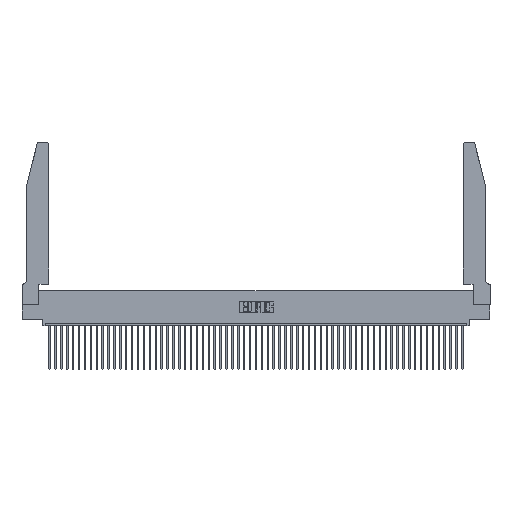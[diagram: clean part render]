
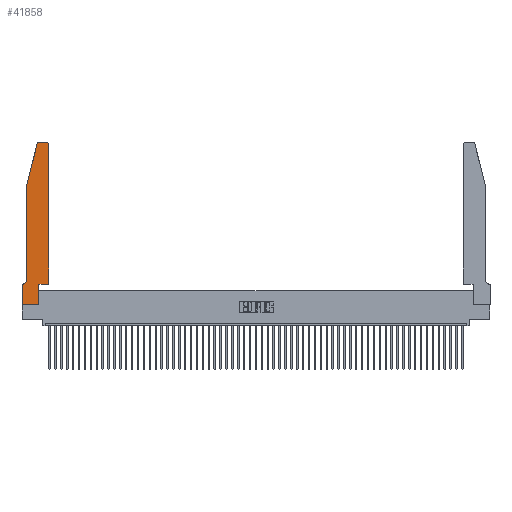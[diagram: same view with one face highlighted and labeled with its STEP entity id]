
A CAD part, top view. The second image highlights one B-rep face of the part: STEP entity #41858.
In plain terms, the highlighted planar face has unit normal (0, 0, 1).
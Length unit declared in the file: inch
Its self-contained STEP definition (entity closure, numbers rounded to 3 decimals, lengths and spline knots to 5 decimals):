
#1388 = CARTESIAN_POINT ( 'NONE',  ( 0.4505, 0.35, 0.37 ) ) ;
#1948 = DIRECTION ( 'NONE',  ( 0., 0., 1. ) ) ;
#2347 = CARTESIAN_POINT ( 'NONE',  ( 0., 0.35, 0.37 ) ) ;
#2770 = DIRECTION ( 'NONE',  ( 0., -1., 0. ) ) ;
#3745 = EDGE_CURVE ( 'NONE', #12074, #40353, #35902, .T. ) ;
#3822 = EDGE_LOOP ( 'NONE', ( #51862, #30141, #5879, #22489, #43303, #23899, #53336, #4882, #50175, #13437, #8664, #28840 ) ) ;
#4216 = DIRECTION ( 'NONE',  ( -0.239, -0.971, 0. ) ) ;
#4882 = ORIENTED_EDGE ( 'NONE', *, *, #9215, .T. ) ;
#5189 = LINE ( 'NONE', #21240, #26146 ) ;
#5588 = DIRECTION ( 'NONE',  ( -1., 0., 0. ) ) ;
#5879 = ORIENTED_EDGE ( 'NONE', *, *, #35239, .T. ) ;
#6450 = DIRECTION ( 'NONE',  ( -1., 0., 0. ) ) ;
#7061 = CARTESIAN_POINT ( 'NONE',  ( 0., 0., 0.37 ) ) ;
#8207 = LINE ( 'NONE', #7061, #25242 ) ;
#8257 = CIRCLE ( 'NONE', #15924, 0.07 ) ;
#8345 = CARTESIAN_POINT ( 'NONE',  ( 0.2605, 2.75, 0.37 ) ) ;
#8349 = CARTESIAN_POINT ( 'NONE',  ( 0.0755, 2., 0.37 ) ) ;
#8664 = ORIENTED_EDGE ( 'NONE', *, *, #11363, .T. ) ;
#9215 = EDGE_CURVE ( 'NONE', #18021, #46392, #42642, .T. ) ;
#9632 = DIRECTION ( 'NONE',  ( -1., 0., 0. ) ) ;
#10883 = VECTOR ( 'NONE', #48942, 39.37008 ) ;
#11363 = EDGE_CURVE ( 'NONE', #18905, #37915, #25783, .T. ) ;
#11902 = FACE_OUTER_BOUND ( 'NONE', #3822, .T. ) ;
#12074 = VERTEX_POINT ( 'NONE', #8349 ) ;
#13437 = ORIENTED_EDGE ( 'NONE', *, *, #32538, .T. ) ;
#13630 = CARTESIAN_POINT ( 'NONE',  ( 0.0055, 0.35, 0.37 ) ) ;
#13858 = DIRECTION ( 'NONE',  ( 0., 0., -1. ) ) ;
#15619 = AXIS2_PLACEMENT_3D ( 'NONE', #2347, #1948, #40471 ) ;
#15924 = AXIS2_PLACEMENT_3D ( 'NONE', #34773, #13858, #9632 ) ;
#18021 = VERTEX_POINT ( 'NONE', #51473 ) ;
#18905 = VERTEX_POINT ( 'NONE', #1388 ) ;
#19006 = CARTESIAN_POINT ( 'NONE',  ( 0.284, 2.75, 0.37 ) ) ;
#19090 = CARTESIAN_POINT ( 'NONE',  ( 0.0755, 0.35, 0.37 ) ) ;
#19500 = VERTEX_POINT ( 'NONE', #28431 ) ;
#20031 = EDGE_CURVE ( 'NONE', #39617, #21007, #28667, .T. ) ;
#20418 = DIRECTION ( 'NONE',  ( 1., 0., 0. ) ) ;
#20900 = VECTOR ( 'NONE', #33370, 39.37008 ) ;
#21007 = VERTEX_POINT ( 'NONE', #31247 ) ;
#21132 = CIRCLE ( 'NONE', #23765, 0.03 ) ;
#21152 = VERTEX_POINT ( 'NONE', #13630 ) ;
#21240 = CARTESIAN_POINT ( 'NONE',  ( 0.0755, 2., 0.37 ) ) ;
#21683 = EDGE_CURVE ( 'NONE', #19500, #18021, #8207, .T. ) ;
#22460 = CARTESIAN_POINT ( 'NONE',  ( 0.2865, 0.35, 0.37 ) ) ;
#22489 = ORIENTED_EDGE ( 'NONE', *, *, #3745, .T. ) ;
#22784 = LINE ( 'NONE', #22460, #52374 ) ;
#23283 = DIRECTION ( 'NONE',  ( 0., 1., 0. ) ) ;
#23765 = AXIS2_PLACEMENT_3D ( 'NONE', #37857, #33274, #20418 ) ;
#23769 = CARTESIAN_POINT ( 'NONE',  ( 0.2865, 0.35, 0.37 ) ) ;
#23899 = ORIENTED_EDGE ( 'NONE', *, *, #48974, .T. ) ;
#25242 = VECTOR ( 'NONE', #2770, 39.37008 ) ;
#25735 = LINE ( 'NONE', #8345, #48185 ) ;
#25783 = LINE ( 'NONE', #36173, #34985 ) ;
#26146 = VECTOR ( 'NONE', #4216, 39.37008 ) ;
#26509 = VECTOR ( 'NONE', #6450, 39.37008 ) ;
#26691 = CARTESIAN_POINT ( 'NONE',  ( 0.4205, 2.75, 0.37 ) ) ;
#28431 = CARTESIAN_POINT ( 'NONE',  ( 0., 0.35, 0.37 ) ) ;
#28667 = CIRCLE ( 'NONE', #48745, 0.03 ) ;
#28755 = VERTEX_POINT ( 'NONE', #26691 ) ;
#28840 = ORIENTED_EDGE ( 'NONE', *, *, #46699, .T. ) ;
#29139 = EDGE_CURVE ( 'NONE', #40353, #21152, #8257, .T. ) ;
#29727 = EDGE_CURVE ( 'NONE', #28755, #39617, #25735, .T. ) ;
#30047 = DIRECTION ( 'NONE',  ( 1., 0., 0. ) ) ;
#30141 = ORIENTED_EDGE ( 'NONE', *, *, #20031, .T. ) ;
#30896 = CARTESIAN_POINT ( 'NONE',  ( 0.284, 2.72, 0.37 ) ) ;
#31247 = CARTESIAN_POINT ( 'NONE',  ( 0.25487, 2.72718, 0.37 ) ) ;
#31370 = LINE ( 'NONE', #38742, #42628 ) ;
#32538 = EDGE_CURVE ( 'NONE', #52554, #18905, #31370, .T. ) ;
#32606 = CARTESIAN_POINT ( 'NONE',  ( 0.2865, 0., 0.37 ) ) ;
#32935 = EDGE_CURVE ( 'NONE', #46392, #52554, #22784, .T. ) ;
#33179 = CARTESIAN_POINT ( 'NONE',  ( 0., 0., 0.37 ) ) ;
#33274 = DIRECTION ( 'NONE',  ( 0., 0., 1. ) ) ;
#33370 = DIRECTION ( 'NONE',  ( 1., 0., 0. ) ) ;
#34773 = CARTESIAN_POINT ( 'NONE',  ( 0.0055, 0.42, 0.37 ) ) ;
#34985 = VECTOR ( 'NONE', #23283, 39.37008 ) ;
#35239 = EDGE_CURVE ( 'NONE', #21007, #12074, #5189, .T. ) ;
#35902 = LINE ( 'NONE', #39939, #10883 ) ;
#36002 = PLANE ( 'NONE',  #15619 ) ;
#36173 = CARTESIAN_POINT ( 'NONE',  ( 0.4505, 0.35, 0.37 ) ) ;
#37857 = CARTESIAN_POINT ( 'NONE',  ( 0.4205, 2.72, 0.37 ) ) ;
#37915 = VERTEX_POINT ( 'NONE', #45299 ) ;
#38742 = CARTESIAN_POINT ( 'NONE',  ( 0.4505, 0.35, 0.37 ) ) ;
#39617 = VERTEX_POINT ( 'NONE', #19006 ) ;
#39939 = CARTESIAN_POINT ( 'NONE',  ( 0.0755, 2., 0.37 ) ) ;
#39988 = DIRECTION ( 'NONE',  ( 0., 0., 1. ) ) ;
#40353 = VERTEX_POINT ( 'NONE', #45015 ) ;
#40471 = DIRECTION ( 'NONE',  ( 1., 0., 0. ) ) ;
#41858 = ADVANCED_FACE ( 'NONE', ( #11902 ), #36002, .T. ) ;
#42628 = VECTOR ( 'NONE', #30047, 39.37008 ) ;
#42642 = LINE ( 'NONE', #33179, #20900 ) ;
#43050 = LINE ( 'NONE', #19090, #26509 ) ;
#43303 = ORIENTED_EDGE ( 'NONE', *, *, #29139, .T. ) ;
#45015 = CARTESIAN_POINT ( 'NONE',  ( 0.0755, 0.42, 0.37 ) ) ;
#45299 = CARTESIAN_POINT ( 'NONE',  ( 0.4505, 2.72, 0.37 ) ) ;
#46392 = VERTEX_POINT ( 'NONE', #32606 ) ;
#46699 = EDGE_CURVE ( 'NONE', #37915, #28755, #21132, .T. ) ;
#48185 = VECTOR ( 'NONE', #5588, 39.37008 ) ;
#48615 = DIRECTION ( 'NONE',  ( 1., 0., 0. ) ) ;
#48745 = AXIS2_PLACEMENT_3D ( 'NONE', #30896, #39988, #48615 ) ;
#48942 = DIRECTION ( 'NONE',  ( 0., -1., 0. ) ) ;
#48974 = EDGE_CURVE ( 'NONE', #21152, #19500, #43050, .T. ) ;
#50175 = ORIENTED_EDGE ( 'NONE', *, *, #32935, .T. ) ;
#51473 = CARTESIAN_POINT ( 'NONE',  ( 0., 0., 0.37 ) ) ;
#51862 = ORIENTED_EDGE ( 'NONE', *, *, #29727, .T. ) ;
#51873 = DIRECTION ( 'NONE',  ( 0., 1., 0. ) ) ;
#52374 = VECTOR ( 'NONE', #51873, 39.37008 ) ;
#52554 = VERTEX_POINT ( 'NONE', #23769 ) ;
#53336 = ORIENTED_EDGE ( 'NONE', *, *, #21683, .T. ) ;
